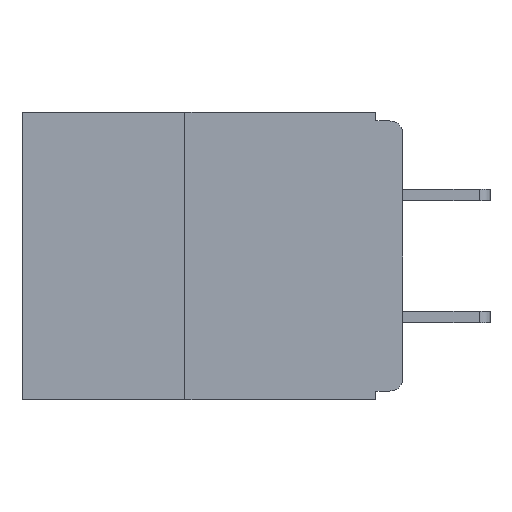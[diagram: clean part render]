
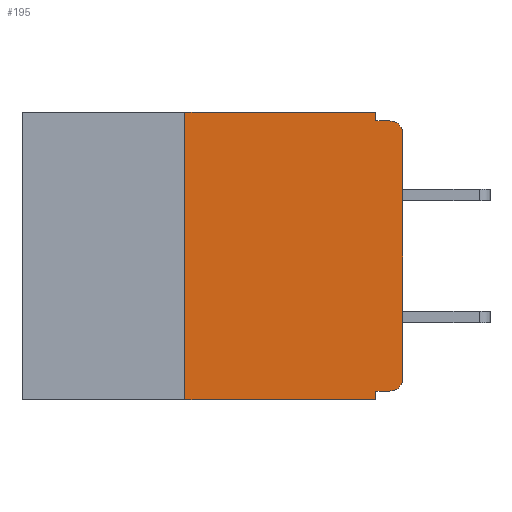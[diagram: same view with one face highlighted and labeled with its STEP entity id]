
A CAD part, left-side view. The second image highlights one B-rep face of the part: STEP entity #195.
In plain terms, the highlighted planar face has unit normal (-1, 0, 0).
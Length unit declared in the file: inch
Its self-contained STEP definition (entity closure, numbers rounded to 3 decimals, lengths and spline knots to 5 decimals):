
#31 = CARTESIAN_POINT ( 'NONE',  ( 0., 0.437, 0. ) ) ;
#195 = ADVANCED_FACE ( 'NONE', ( #5626 ), #6799, .F. ) ;
#285 = CARTESIAN_POINT ( 'NONE',  ( 0., 0.25, -0.33 ) ) ;
#300 = DIRECTION ( 'NONE',  ( 0., -1., 0. ) ) ;
#375 = VECTOR ( 'NONE', #5683, 39.37008 ) ;
#786 = LINE ( 'NONE', #2741, #6742 ) ;
#794 = LINE ( 'NONE', #10855, #375 ) ;
#1079 = ORIENTED_EDGE ( 'NONE', *, *, #6847, .T. ) ;
#1570 = LINE ( 'NONE', #11839, #1589 ) ;
#1589 = VECTOR ( 'NONE', #11906, 39.37008 ) ;
#1838 = VECTOR ( 'NONE', #3683, 39.37008 ) ;
#1866 = EDGE_CURVE ( 'NONE', #5469, #4069, #7235, .T. ) ;
#1902 = LINE ( 'NONE', #3592, #1838 ) ;
#2047 = VERTEX_POINT ( 'NONE', #6866 ) ;
#2135 = DIRECTION ( 'NONE',  ( 0., 0., 1. ) ) ;
#2290 = ORIENTED_EDGE ( 'NONE', *, *, #7597, .F. ) ;
#2398 = EDGE_CURVE ( 'NONE', #4081, #6237, #794, .T. ) ;
#2723 = CARTESIAN_POINT ( 'NONE',  ( 0., 0., 0. ) ) ;
#2741 = CARTESIAN_POINT ( 'NONE',  ( 0., 0.031, 0. ) ) ;
#2828 = DIRECTION ( 'NONE',  ( 0., 0., -1. ) ) ;
#3030 = ORIENTED_EDGE ( 'NONE', *, *, #2398, .F. ) ;
#3149 = ORIENTED_EDGE ( 'NONE', *, *, #11024, .F. ) ;
#3592 = CARTESIAN_POINT ( 'NONE',  ( 0., 0., -0.32 ) ) ;
#3683 = DIRECTION ( 'NONE',  ( 0., 1., 0. ) ) ;
#3724 = ORIENTED_EDGE ( 'NONE', *, *, #9095, .F. ) ;
#3839 = ORIENTED_EDGE ( 'NONE', *, *, #5812, .T. ) ;
#3862 = CARTESIAN_POINT ( 'NONE',  ( 0., 0.015, -0.01 ) ) ;
#3975 = ORIENTED_EDGE ( 'NONE', *, *, #8669, .T. ) ;
#4069 = VERTEX_POINT ( 'NONE', #9299 ) ;
#4081 = VERTEX_POINT ( 'NONE', #11540 ) ;
#4322 = LINE ( 'NONE', #2723, #4574 ) ;
#4478 = EDGE_LOOP ( 'NONE', ( #3839, #3975, #10296, #2290, #3724, #5536, #1079, #3030, #3149, #8986 ) ) ;
#4574 = VECTOR ( 'NONE', #2135, 39.37008 ) ;
#5352 = AXIS2_PLACEMENT_3D ( 'NONE', #8961, #7650, #7306 ) ;
#5469 = VERTEX_POINT ( 'NONE', #7754 ) ;
#5536 = ORIENTED_EDGE ( 'NONE', *, *, #8690, .F. ) ;
#5563 = VERTEX_POINT ( 'NONE', #6602 ) ;
#5626 = FACE_OUTER_BOUND ( 'NONE', #4478, .T. ) ;
#5683 = DIRECTION ( 'NONE',  ( 0., 0., -1. ) ) ;
#5812 = EDGE_CURVE ( 'NONE', #4069, #5563, #4322, .T. ) ;
#5858 = VECTOR ( 'NONE', #10375, 39.37008 ) ;
#6237 = VERTEX_POINT ( 'NONE', #6665 ) ;
#6302 = LINE ( 'NONE', #10391, #5858 ) ;
#6581 = DIRECTION ( 'NONE',  ( 0., 0., -1. ) ) ;
#6602 = CARTESIAN_POINT ( 'NONE',  ( 0., 0., -0.025 ) ) ;
#6665 = CARTESIAN_POINT ( 'NONE',  ( 0., 0.031, -0.33 ) ) ;
#6715 = DIRECTION ( 'NONE',  ( 1., 0., 0. ) ) ;
#6742 = VECTOR ( 'NONE', #2828, 39.37008 ) ;
#6799 = PLANE ( 'NONE',  #10435 ) ;
#6810 = CARTESIAN_POINT ( 'NONE',  ( 0., 0.031, 0. ) ) ;
#6847 = EDGE_CURVE ( 'NONE', #9089, #6237, #6302, .T. ) ;
#6866 = CARTESIAN_POINT ( 'NONE',  ( 0., 0.25, 0. ) ) ;
#7235 = CIRCLE ( 'NONE', #5352, 0.015 ) ;
#7256 = VERTEX_POINT ( 'NONE', #6810 ) ;
#7306 = DIRECTION ( 'NONE',  ( 0., 0., -1. ) ) ;
#7542 = VERTEX_POINT ( 'NONE', #3862 ) ;
#7597 = EDGE_CURVE ( 'NONE', #7256, #8150, #786, .T. ) ;
#7650 = DIRECTION ( 'NONE',  ( -1., 0., 0. ) ) ;
#7754 = CARTESIAN_POINT ( 'NONE',  ( 0., 0.015, -0.32 ) ) ;
#8069 = EDGE_CURVE ( 'NONE', #8150, #7542, #1570, .T. ) ;
#8150 = VERTEX_POINT ( 'NONE', #9480 ) ;
#8669 = EDGE_CURVE ( 'NONE', #5563, #7542, #10814, .T. ) ;
#8690 = EDGE_CURVE ( 'NONE', #9089, #2047, #10734, .T. ) ;
#8961 = CARTESIAN_POINT ( 'NONE',  ( 0., 0.015, -0.305 ) ) ;
#8986 = ORIENTED_EDGE ( 'NONE', *, *, #1866, .T. ) ;
#9089 = VERTEX_POINT ( 'NONE', #285 ) ;
#9095 = EDGE_CURVE ( 'NONE', #2047, #7256, #9234, .T. ) ;
#9205 = VECTOR ( 'NONE', #300, 39.37008 ) ;
#9234 = LINE ( 'NONE', #31, #9205 ) ;
#9299 = CARTESIAN_POINT ( 'NONE',  ( 0., 0., -0.305 ) ) ;
#9480 = CARTESIAN_POINT ( 'NONE',  ( 0., 0.031, -0.01 ) ) ;
#9786 = CARTESIAN_POINT ( 'NONE',  ( 0., 0.437, 0. ) ) ;
#10296 = ORIENTED_EDGE ( 'NONE', *, *, #8069, .F. ) ;
#10375 = DIRECTION ( 'NONE',  ( 0., -1., 0. ) ) ;
#10391 = CARTESIAN_POINT ( 'NONE',  ( 0., 0.437, -0.33 ) ) ;
#10435 = AXIS2_PLACEMENT_3D ( 'NONE', #9786, #6715, #6581 ) ;
#10717 = VECTOR ( 'NONE', #11002, 39.37008 ) ;
#10734 = LINE ( 'NONE', #10982, #10717 ) ;
#10814 = CIRCLE ( 'NONE', #11217, 0.015 ) ;
#10855 = CARTESIAN_POINT ( 'NONE',  ( 0., 0.031, -0.33 ) ) ;
#10982 = CARTESIAN_POINT ( 'NONE',  ( 0., 0.25, -0.33 ) ) ;
#11002 = DIRECTION ( 'NONE',  ( 0., 0., 1. ) ) ;
#11024 = EDGE_CURVE ( 'NONE', #5469, #4081, #1902, .T. ) ;
#11125 = DIRECTION ( 'NONE',  ( 0., 0., -1. ) ) ;
#11154 = DIRECTION ( 'NONE',  ( -1., 0., 0. ) ) ;
#11216 = CARTESIAN_POINT ( 'NONE',  ( 0., 0.015, -0.025 ) ) ;
#11217 = AXIS2_PLACEMENT_3D ( 'NONE', #11216, #11154, #11125 ) ;
#11540 = CARTESIAN_POINT ( 'NONE',  ( 0., 0.031, -0.32 ) ) ;
#11839 = CARTESIAN_POINT ( 'NONE',  ( 0., 0., -0.01 ) ) ;
#11906 = DIRECTION ( 'NONE',  ( 0., -1., 0. ) ) ;
